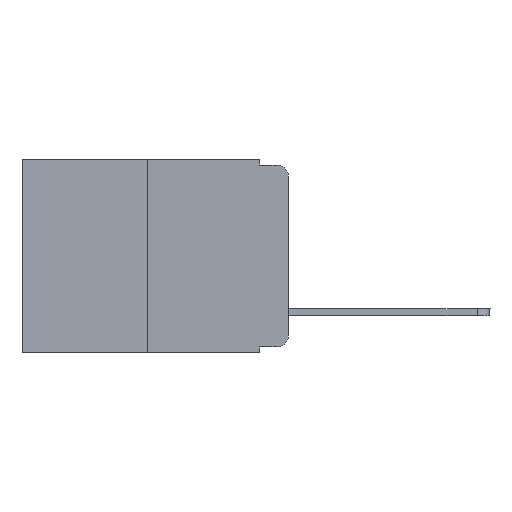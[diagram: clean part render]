
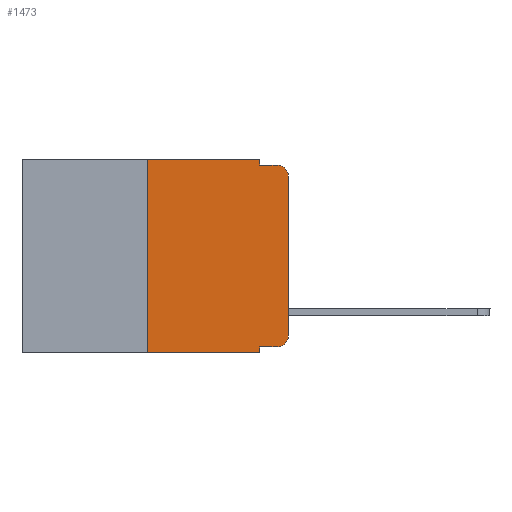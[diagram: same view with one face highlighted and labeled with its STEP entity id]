
A CAD part, left-side view. The second image highlights one B-rep face of the part: STEP entity #1473.
In plain terms, the highlighted planar face has unit normal (-1, 0, 0).
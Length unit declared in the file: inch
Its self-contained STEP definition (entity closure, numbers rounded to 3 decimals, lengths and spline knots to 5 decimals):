
#143 = ORIENTED_EDGE ( 'NONE', *, *, #17219, .F. ) ;
#206 = CARTESIAN_POINT ( 'NONE',  ( 0., 0.051, 0. ) ) ;
#296 = VECTOR ( 'NONE', #19081, 39.37008 ) ;
#534 = AXIS2_PLACEMENT_3D ( 'NONE', #12035, #11697, #18801 ) ;
#752 = LINE ( 'NONE', #14228, #20532 ) ;
#783 = LINE ( 'NONE', #14594, #12132 ) ;
#791 = VERTEX_POINT ( 'NONE', #9491 ) ;
#866 = EDGE_CURVE ( 'NONE', #13377, #791, #783, .T. ) ;
#896 = CIRCLE ( 'NONE', #534, 0.02 ) ;
#1326 = CARTESIAN_POINT ( 'NONE',  ( 0., 0.051, 0. ) ) ;
#1473 = ADVANCED_FACE ( 'NONE', ( #12005 ), #3510, .F. ) ;
#1655 = VECTOR ( 'NONE', #10492, 39.37008 ) ;
#1770 = CARTESIAN_POINT ( 'NONE',  ( 0., 0., -0.313 ) ) ;
#1938 = LINE ( 'NONE', #15193, #8256 ) ;
#2935 = CARTESIAN_POINT ( 'NONE',  ( 0., 0.051, -0.333 ) ) ;
#3342 = VERTEX_POINT ( 'NONE', #20408 ) ;
#3510 = PLANE ( 'NONE',  #7529 ) ;
#4097 = EDGE_CURVE ( 'NONE', #11739, #21399, #896, .T. ) ;
#4348 = DIRECTION ( 'NONE',  ( 0., -1., 0. ) ) ;
#5460 = EDGE_LOOP ( 'NONE', ( #14845, #20668, #143, #14546, #16854, #16774, #19382, #9400, #18023, #9552 ) ) ;
#6182 = CARTESIAN_POINT ( 'NONE',  ( 0., 0.473, -0.343 ) ) ;
#6331 = CARTESIAN_POINT ( 'NONE',  ( 0., 0.25, 0. ) ) ;
#6416 = VERTEX_POINT ( 'NONE', #18272 ) ;
#6655 = LINE ( 'NONE', #1326, #7137 ) ;
#7021 = EDGE_CURVE ( 'NONE', #12717, #11739, #752, .T. ) ;
#7079 = DIRECTION ( 'NONE',  ( 1., 0., 0. ) ) ;
#7137 = VECTOR ( 'NONE', #21704, 39.37008 ) ;
#7398 = CARTESIAN_POINT ( 'NONE',  ( 0., 0.25, 0. ) ) ;
#7529 = AXIS2_PLACEMENT_3D ( 'NONE', #15665, #7079, #17429 ) ;
#7794 = VERTEX_POINT ( 'NONE', #13822 ) ;
#7835 = DIRECTION ( 'NONE',  ( 0., 0., -1. ) ) ;
#7922 = VERTEX_POINT ( 'NONE', #19917 ) ;
#8256 = VECTOR ( 'NONE', #18519, 39.37008 ) ;
#8353 = VECTOR ( 'NONE', #21419, 39.37008 ) ;
#8827 = VECTOR ( 'NONE', #13162, 39.37008 ) ;
#8983 = CIRCLE ( 'NONE', #9348, 0.02 ) ;
#8991 = EDGE_CURVE ( 'NONE', #12717, #3342, #15376, .T. ) ;
#9348 = AXIS2_PLACEMENT_3D ( 'NONE', #19494, #9402, #7835 ) ;
#9400 = ORIENTED_EDGE ( 'NONE', *, *, #8991, .F. ) ;
#9402 = DIRECTION ( 'NONE',  ( -1., 0., 0. ) ) ;
#9478 = EDGE_CURVE ( 'NONE', #6416, #3342, #15875, .T. ) ;
#9491 = CARTESIAN_POINT ( 'NONE',  ( 0., 0.051, 0. ) ) ;
#9552 = ORIENTED_EDGE ( 'NONE', *, *, #4097, .T. ) ;
#10066 = EDGE_CURVE ( 'NONE', #21399, #7794, #21611, .T. ) ;
#10492 = DIRECTION ( 'NONE',  ( 0., 0., -1. ) ) ;
#11697 = DIRECTION ( 'NONE',  ( -1., 0., 0. ) ) ;
#11739 = VERTEX_POINT ( 'NONE', #21252 ) ;
#12005 = FACE_OUTER_BOUND ( 'NONE', #5460, .T. ) ;
#12035 = CARTESIAN_POINT ( 'NONE',  ( 0., 0.02, -0.313 ) ) ;
#12132 = VECTOR ( 'NONE', #4348, 39.37008 ) ;
#12543 = EDGE_CURVE ( 'NONE', #6416, #13377, #17310, .T. ) ;
#12717 = VERTEX_POINT ( 'NONE', #2935 ) ;
#13162 = DIRECTION ( 'NONE',  ( 0., 0., 1. ) ) ;
#13377 = VERTEX_POINT ( 'NONE', #6331 ) ;
#13822 = CARTESIAN_POINT ( 'NONE',  ( 0., 0., -0.03 ) ) ;
#14228 = CARTESIAN_POINT ( 'NONE',  ( 0., 0.051, -0.333 ) ) ;
#14512 = CARTESIAN_POINT ( 'NONE',  ( 0., 0.051, -0.01 ) ) ;
#14546 = ORIENTED_EDGE ( 'NONE', *, *, #15834, .F. ) ;
#14594 = CARTESIAN_POINT ( 'NONE',  ( 0., 0.473, 0. ) ) ;
#14845 = ORIENTED_EDGE ( 'NONE', *, *, #10066, .T. ) ;
#15193 = CARTESIAN_POINT ( 'NONE',  ( 0., 0.051, -0.01 ) ) ;
#15376 = LINE ( 'NONE', #206, #1655 ) ;
#15665 = CARTESIAN_POINT ( 'NONE',  ( 0., 0.473, 0. ) ) ;
#15834 = EDGE_CURVE ( 'NONE', #791, #18887, #6655, .T. ) ;
#15875 = LINE ( 'NONE', #6182, #8353 ) ;
#16774 = ORIENTED_EDGE ( 'NONE', *, *, #12543, .F. ) ;
#16854 = ORIENTED_EDGE ( 'NONE', *, *, #866, .F. ) ;
#17219 = EDGE_CURVE ( 'NONE', #18887, #7922, #1938, .T. ) ;
#17310 = LINE ( 'NONE', #7398, #296 ) ;
#17429 = DIRECTION ( 'NONE',  ( 0., 0., -1. ) ) ;
#17554 = EDGE_CURVE ( 'NONE', #7794, #7922, #8983, .T. ) ;
#18023 = ORIENTED_EDGE ( 'NONE', *, *, #7021, .T. ) ;
#18160 = CARTESIAN_POINT ( 'NONE',  ( 0., 0., 0. ) ) ;
#18272 = CARTESIAN_POINT ( 'NONE',  ( 0., 0.25, -0.343 ) ) ;
#18519 = DIRECTION ( 'NONE',  ( 0., -1., 0. ) ) ;
#18801 = DIRECTION ( 'NONE',  ( 0., 0., -1. ) ) ;
#18887 = VERTEX_POINT ( 'NONE', #14512 ) ;
#19081 = DIRECTION ( 'NONE',  ( 0., 0., 1. ) ) ;
#19336 = DIRECTION ( 'NONE',  ( 0., -1., 0. ) ) ;
#19382 = ORIENTED_EDGE ( 'NONE', *, *, #9478, .T. ) ;
#19494 = CARTESIAN_POINT ( 'NONE',  ( 0., 0.02, -0.03 ) ) ;
#19917 = CARTESIAN_POINT ( 'NONE',  ( 0., 0.02, -0.01 ) ) ;
#20408 = CARTESIAN_POINT ( 'NONE',  ( 0., 0.051, -0.343 ) ) ;
#20532 = VECTOR ( 'NONE', #19336, 39.37008 ) ;
#20668 = ORIENTED_EDGE ( 'NONE', *, *, #17554, .T. ) ;
#21252 = CARTESIAN_POINT ( 'NONE',  ( 0., 0.02, -0.333 ) ) ;
#21399 = VERTEX_POINT ( 'NONE', #1770 ) ;
#21419 = DIRECTION ( 'NONE',  ( 0., -1., 0. ) ) ;
#21611 = LINE ( 'NONE', #18160, #8827 ) ;
#21704 = DIRECTION ( 'NONE',  ( 0., 0., -1. ) ) ;
